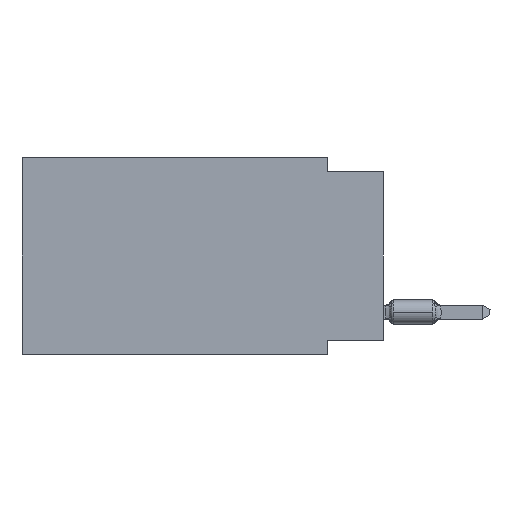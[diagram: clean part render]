
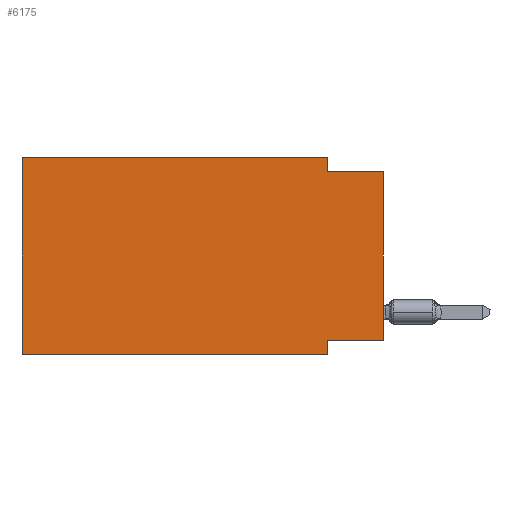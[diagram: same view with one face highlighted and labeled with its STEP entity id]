
A CAD part, left-side view. The second image highlights one B-rep face of the part: STEP entity #6175.
In plain terms, the highlighted planar face has unit normal (-1, 0, 0).
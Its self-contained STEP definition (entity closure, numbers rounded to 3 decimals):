
#339 = DIRECTION ( 'NONE',  ( 0., 0., -1. ) ) ;
#369 = DIRECTION ( 'NONE',  ( 0., 0., -1. ) ) ;
#851 = DIRECTION ( 'NONE',  ( 0., 0., -1. ) ) ;
#1698 = ORIENTED_EDGE ( 'NONE', *, *, #8208, .F. ) ;
#1902 = DIRECTION ( 'NONE',  ( 0., -1., 0. ) ) ;
#2020 = VERTEX_POINT ( 'NONE', #3105 ) ;
#2022 = VECTOR ( 'NONE', #27100, 1000. ) ;
#2137 = VECTOR ( 'NONE', #16343, 1000. ) ;
#2677 = ORIENTED_EDGE ( 'NONE', *, *, #5753, .T. ) ;
#2863 = LINE ( 'NONE', #6079, #8778 ) ;
#3053 = CARTESIAN_POINT ( 'NONE',  ( 0., 2.54, -8.89 ) ) ;
#3084 = CARTESIAN_POINT ( 'NONE',  ( 0., 0., -0.635 ) ) ;
#3105 = CARTESIAN_POINT ( 'NONE',  ( 0., 16.383, 0. ) ) ;
#3674 = VECTOR ( 'NONE', #1902, 1000. ) ;
#4249 = LINE ( 'NONE', #17214, #2022 ) ;
#4381 = VERTEX_POINT ( 'NONE', #20646 ) ;
#5753 = EDGE_CURVE ( 'NONE', #20837, #11826, #27137, .T. ) ;
#5874 = VERTEX_POINT ( 'NONE', #6046 ) ;
#6046 = CARTESIAN_POINT ( 'NONE',  ( 0., 2.54, -0.635 ) ) ;
#6079 = CARTESIAN_POINT ( 'NONE',  ( 0., 16.383, 0. ) ) ;
#6175 = ADVANCED_FACE ( 'NONE', ( #17867 ), #12545, .F. ) ;
#6508 = CARTESIAN_POINT ( 'NONE',  ( 0., 0., 0. ) ) ;
#6750 = LINE ( 'NONE', #8709, #2137 ) ;
#7432 = VERTEX_POINT ( 'NONE', #26496 ) ;
#8208 = EDGE_CURVE ( 'NONE', #5874, #17086, #26547, .T. ) ;
#8709 = CARTESIAN_POINT ( 'NONE',  ( 0., 0., -8.255 ) ) ;
#8778 = VECTOR ( 'NONE', #12769, 1000. ) ;
#9029 = EDGE_CURVE ( 'NONE', #14767, #7432, #6750, .T. ) ;
#9371 = EDGE_CURVE ( 'NONE', #14767, #17086, #29352, .T. ) ;
#9498 = AXIS2_PLACEMENT_3D ( 'NONE', #17703, #20126, #339 ) ;
#9543 = ORIENTED_EDGE ( 'NONE', *, *, #9029, .F. ) ;
#11826 = VERTEX_POINT ( 'NONE', #3053 ) ;
#11943 = CARTESIAN_POINT ( 'NONE',  ( 0., 0., -8.255 ) ) ;
#12545 = PLANE ( 'NONE',  #9498 ) ;
#12731 = CARTESIAN_POINT ( 'NONE',  ( 0., 16.383, -8.89 ) ) ;
#12769 = DIRECTION ( 'NONE',  ( 0., 0., 1. ) ) ;
#13353 = CARTESIAN_POINT ( 'NONE',  ( 0., 2.54, 0. ) ) ;
#14127 = ORIENTED_EDGE ( 'NONE', *, *, #14304, .F. ) ;
#14304 = EDGE_CURVE ( 'NONE', #7432, #11826, #23066, .T. ) ;
#14767 = VERTEX_POINT ( 'NONE', #11943 ) ;
#16343 = DIRECTION ( 'NONE',  ( 0., 1., 0. ) ) ;
#16572 = DIRECTION ( 'NONE',  ( 0., 0., 1. ) ) ;
#17086 = VERTEX_POINT ( 'NONE', #3084 ) ;
#17214 = CARTESIAN_POINT ( 'NONE',  ( 0., 16.383, 0. ) ) ;
#17619 = ORIENTED_EDGE ( 'NONE', *, *, #20914, .F. ) ;
#17703 = CARTESIAN_POINT ( 'NONE',  ( 0., 16.383, 0. ) ) ;
#17867 = FACE_OUTER_BOUND ( 'NONE', #28466, .T. ) ;
#18903 = ORIENTED_EDGE ( 'NONE', *, *, #9371, .T. ) ;
#20126 = DIRECTION ( 'NONE',  ( 1., 0., 0. ) ) ;
#20646 = CARTESIAN_POINT ( 'NONE',  ( 0., 2.54, 0. ) ) ;
#20837 = VERTEX_POINT ( 'NONE', #29272 ) ;
#20914 = EDGE_CURVE ( 'NONE', #4381, #5874, #30211, .T. ) ;
#21038 = CARTESIAN_POINT ( 'NONE',  ( 0., 0., -0.635 ) ) ;
#21233 = ORIENTED_EDGE ( 'NONE', *, *, #23247, .F. ) ;
#21379 = VECTOR ( 'NONE', #369, 1000. ) ;
#22764 = EDGE_CURVE ( 'NONE', #2020, #4381, #4249, .T. ) ;
#23066 = LINE ( 'NONE', #28085, #30170 ) ;
#23247 = EDGE_CURVE ( 'NONE', #20837, #2020, #2863, .T. ) ;
#23317 = VECTOR ( 'NONE', #16572, 1000. ) ;
#24100 = ORIENTED_EDGE ( 'NONE', *, *, #22764, .F. ) ;
#26496 = CARTESIAN_POINT ( 'NONE',  ( 0., 2.54, -8.255 ) ) ;
#26547 = LINE ( 'NONE', #21038, #3674 ) ;
#27100 = DIRECTION ( 'NONE',  ( 0., -1., 0. ) ) ;
#27137 = LINE ( 'NONE', #12731, #31705 ) ;
#28085 = CARTESIAN_POINT ( 'NONE',  ( 0., 2.54, -8.89 ) ) ;
#28466 = EDGE_LOOP ( 'NONE', ( #18903, #1698, #17619, #24100, #21233, #2677, #14127, #9543 ) ) ;
#29272 = CARTESIAN_POINT ( 'NONE',  ( 0., 16.383, -8.89 ) ) ;
#29352 = LINE ( 'NONE', #6508, #23317 ) ;
#29721 = DIRECTION ( 'NONE',  ( 0., -1., 0. ) ) ;
#30170 = VECTOR ( 'NONE', #851, 1000. ) ;
#30211 = LINE ( 'NONE', #13353, #21379 ) ;
#31705 = VECTOR ( 'NONE', #29721, 1000. ) ;
